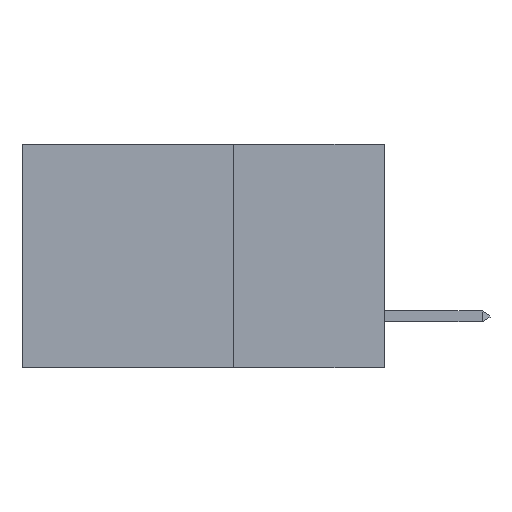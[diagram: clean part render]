
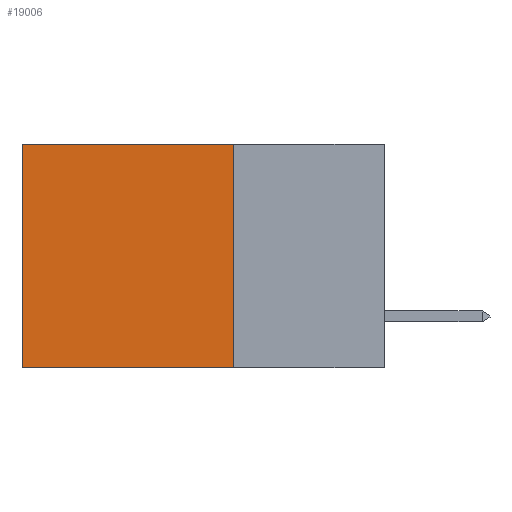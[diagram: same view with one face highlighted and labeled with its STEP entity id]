
A CAD part, left-side view. The second image highlights one B-rep face of the part: STEP entity #19006.
In plain terms, the highlighted planar face has unit normal (-1, 0, 0).
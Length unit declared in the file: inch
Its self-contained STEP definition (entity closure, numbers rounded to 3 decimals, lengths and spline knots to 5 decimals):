
#112 = DIRECTION ( 'NONE',  ( 0., 1., 0. ) ) ;
#687 = VERTEX_POINT ( 'NONE', #17927 ) ;
#801 = CARTESIAN_POINT ( 'NONE',  ( 0.2875, 0.6, 0. ) ) ;
#948 = ORIENTED_EDGE ( 'NONE', *, *, #1027, .T. ) ;
#1027 = EDGE_CURVE ( 'NONE', #7207, #687, #10358, .T. ) ;
#1142 = DIRECTION ( 'NONE',  ( 1., 0., 0. ) ) ;
#1226 = ORIENTED_EDGE ( 'NONE', *, *, #18602, .F. ) ;
#1597 = LINE ( 'NONE', #15822, #18065 ) ;
#3521 = CARTESIAN_POINT ( 'NONE',  ( 0.2875, 0.25, -0.37 ) ) ;
#4751 = LINE ( 'NONE', #15886, #16654 ) ;
#4961 = DIRECTION ( 'NONE',  ( 0., 1., 0. ) ) ;
#6077 = VECTOR ( 'NONE', #17300, 39.37008 ) ;
#6330 = VERTEX_POINT ( 'NONE', #3521 ) ;
#7207 = VERTEX_POINT ( 'NONE', #13254 ) ;
#8230 = DIRECTION ( 'NONE',  ( 0., 0., -1. ) ) ;
#10358 = LINE ( 'NONE', #801, #6077 ) ;
#10581 = CARTESIAN_POINT ( 'NONE',  ( 0.2875, 0.25, 0. ) ) ;
#10745 = FACE_OUTER_BOUND ( 'NONE', #14386, .T. ) ;
#10766 = VECTOR ( 'NONE', #112, 39.37008 ) ;
#12155 = DIRECTION ( 'NONE',  ( 0., 0., -1. ) ) ;
#12860 = EDGE_CURVE ( 'NONE', #17921, #7207, #1597, .T. ) ;
#12913 = EDGE_CURVE ( 'NONE', #17921, #6330, #4751, .T. ) ;
#13254 = CARTESIAN_POINT ( 'NONE',  ( 0.2875, 0.6, 0. ) ) ;
#13326 = ORIENTED_EDGE ( 'NONE', *, *, #12913, .F. ) ;
#14188 = CARTESIAN_POINT ( 'NONE',  ( 0.2875, 0.25, -0.37 ) ) ;
#14386 = EDGE_LOOP ( 'NONE', ( #948, #1226, #13326, #14451 ) ) ;
#14451 = ORIENTED_EDGE ( 'NONE', *, *, #12860, .T. ) ;
#15455 = CARTESIAN_POINT ( 'NONE',  ( 0.2875, 0.25, 0. ) ) ;
#15822 = CARTESIAN_POINT ( 'NONE',  ( 0.2875, 0.25, 0. ) ) ;
#15886 = CARTESIAN_POINT ( 'NONE',  ( 0.2875, 0.25, 0. ) ) ;
#16654 = VECTOR ( 'NONE', #8230, 39.37008 ) ;
#17300 = DIRECTION ( 'NONE',  ( 0., 0., -1. ) ) ;
#17580 = AXIS2_PLACEMENT_3D ( 'NONE', #10581, #1142, #12155 ) ;
#17921 = VERTEX_POINT ( 'NONE', #15455 ) ;
#17927 = CARTESIAN_POINT ( 'NONE',  ( 0.2875, 0.6, -0.37 ) ) ;
#18065 = VECTOR ( 'NONE', #4961, 39.37008 ) ;
#18602 = EDGE_CURVE ( 'NONE', #6330, #687, #18773, .T. ) ;
#18773 = LINE ( 'NONE', #14188, #10766 ) ;
#19006 = ADVANCED_FACE ( 'NONE', ( #10745 ), #19586, .F. ) ;
#19586 = PLANE ( 'NONE',  #17580 ) ;
